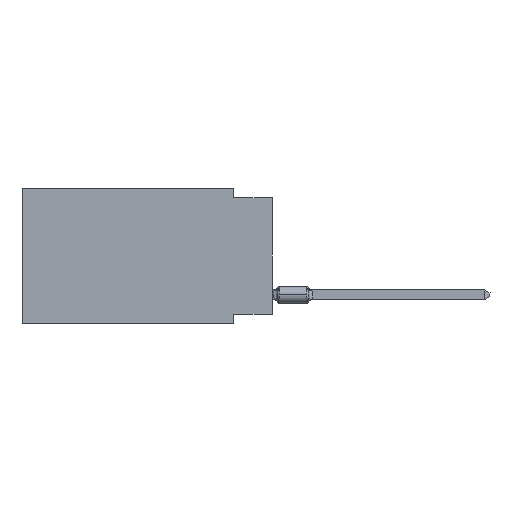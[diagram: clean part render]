
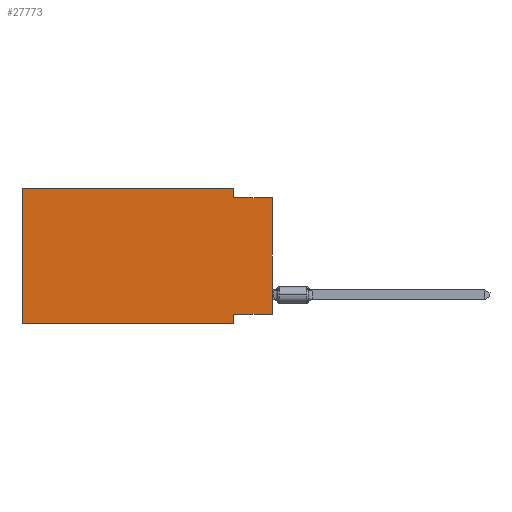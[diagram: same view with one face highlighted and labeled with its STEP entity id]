
A CAD part, left-side view. The second image highlights one B-rep face of the part: STEP entity #27773.
In plain terms, the highlighted planar face has unit normal (-1, 0, 0).
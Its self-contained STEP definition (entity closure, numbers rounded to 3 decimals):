
#157 = ORIENTED_EDGE ( 'NONE', *, *, #20566, .F. ) ;
#1232 = VERTEX_POINT ( 'NONE', #8478 ) ;
#1319 = VERTEX_POINT ( 'NONE', #1795 ) ;
#1593 = EDGE_CURVE ( 'NONE', #19388, #13219, #30711, .T. ) ;
#1795 = CARTESIAN_POINT ( 'NONE',  ( 0., 2.54, -8.255 ) ) ;
#1906 = DIRECTION ( 'NONE',  ( 0., -1., 0. ) ) ;
#2974 = LINE ( 'NONE', #7769, #18852 ) ;
#3166 = CARTESIAN_POINT ( 'NONE',  ( 0., 0., -0.635 ) ) ;
#3700 = LINE ( 'NONE', #13406, #22233 ) ;
#3973 = EDGE_CURVE ( 'NONE', #13219, #11547, #6130, .T. ) ;
#4017 = CARTESIAN_POINT ( 'NONE',  ( 0., 16.383, 0. ) ) ;
#4043 = AXIS2_PLACEMENT_3D ( 'NONE', #4017, #11180, #21385 ) ;
#4394 = LINE ( 'NONE', #12014, #19339 ) ;
#4934 = EDGE_CURVE ( 'NONE', #19388, #9634, #21191, .T. ) ;
#5345 = VERTEX_POINT ( 'NONE', #3166 ) ;
#5811 = VERTEX_POINT ( 'NONE', #7577 ) ;
#6130 = LINE ( 'NONE', #15852, #12876 ) ;
#6335 = CARTESIAN_POINT ( 'NONE',  ( 0., 16.383, 0. ) ) ;
#7226 = LINE ( 'NONE', #22345, #17469 ) ;
#7577 = CARTESIAN_POINT ( 'NONE',  ( 0., 0., -8.255 ) ) ;
#7591 = DIRECTION ( 'NONE',  ( 0., 0., 1. ) ) ;
#7677 = ORIENTED_EDGE ( 'NONE', *, *, #4934, .T. ) ;
#7769 = CARTESIAN_POINT ( 'NONE',  ( 0., 0., 0. ) ) ;
#7908 = CARTESIAN_POINT ( 'NONE',  ( 0., 2.54, -8.89 ) ) ;
#8305 = ORIENTED_EDGE ( 'NONE', *, *, #1593, .F. ) ;
#8478 = CARTESIAN_POINT ( 'NONE',  ( 0., 2.54, -0.635 ) ) ;
#8946 = PLANE ( 'NONE',  #4043 ) ;
#9634 = VERTEX_POINT ( 'NONE', #7908 ) ;
#9698 = EDGE_CURVE ( 'NONE', #5811, #5345, #2974, .T. ) ;
#10855 = DIRECTION ( 'NONE',  ( 0., -1., 0. ) ) ;
#10997 = ORIENTED_EDGE ( 'NONE', *, *, #27568, .F. ) ;
#11180 = DIRECTION ( 'NONE',  ( 1., 0., 0. ) ) ;
#11547 = VERTEX_POINT ( 'NONE', #21206 ) ;
#11580 = VECTOR ( 'NONE', #19209, 1000. ) ;
#12014 = CARTESIAN_POINT ( 'NONE',  ( 0., 2.54, -8.89 ) ) ;
#12876 = VECTOR ( 'NONE', #25576, 1000. ) ;
#13219 = VERTEX_POINT ( 'NONE', #17408 ) ;
#13406 = CARTESIAN_POINT ( 'NONE',  ( 0., 0., -0.635 ) ) ;
#14019 = CARTESIAN_POINT ( 'NONE',  ( 0., 16.383, -8.89 ) ) ;
#14486 = ORIENTED_EDGE ( 'NONE', *, *, #16283, .F. ) ;
#15090 = ORIENTED_EDGE ( 'NONE', *, *, #20014, .F. ) ;
#15160 = DIRECTION ( 'NONE',  ( 0., 0., -1. ) ) ;
#15852 = CARTESIAN_POINT ( 'NONE',  ( 0., 16.383, 0. ) ) ;
#16050 = DIRECTION ( 'NONE',  ( 0., 0., 1. ) ) ;
#16283 = EDGE_CURVE ( 'NONE', #1319, #9634, #4394, .T. ) ;
#17408 = CARTESIAN_POINT ( 'NONE',  ( 0., 16.383, 0. ) ) ;
#17469 = VECTOR ( 'NONE', #15160, 1000. ) ;
#17475 = ORIENTED_EDGE ( 'NONE', *, *, #3973, .F. ) ;
#18744 = LINE ( 'NONE', #28451, #11580 ) ;
#18852 = VECTOR ( 'NONE', #7591, 1000. ) ;
#19062 = CARTESIAN_POINT ( 'NONE',  ( 0., 16.383, -8.89 ) ) ;
#19209 = DIRECTION ( 'NONE',  ( 0., 1., 0. ) ) ;
#19339 = VECTOR ( 'NONE', #21592, 1000. ) ;
#19388 = VERTEX_POINT ( 'NONE', #19062 ) ;
#20014 = EDGE_CURVE ( 'NONE', #1232, #5345, #3700, .T. ) ;
#20566 = EDGE_CURVE ( 'NONE', #5811, #1319, #18744, .T. ) ;
#21071 = FACE_OUTER_BOUND ( 'NONE', #31429, .T. ) ;
#21191 = LINE ( 'NONE', #14019, #28073 ) ;
#21206 = CARTESIAN_POINT ( 'NONE',  ( 0., 2.54, 0. ) ) ;
#21385 = DIRECTION ( 'NONE',  ( 0., 0., -1. ) ) ;
#21592 = DIRECTION ( 'NONE',  ( 0., 0., -1. ) ) ;
#21718 = VECTOR ( 'NONE', #16050, 1000. ) ;
#22233 = VECTOR ( 'NONE', #10855, 1000. ) ;
#22345 = CARTESIAN_POINT ( 'NONE',  ( 0., 2.54, 0. ) ) ;
#25576 = DIRECTION ( 'NONE',  ( 0., -1., 0. ) ) ;
#27174 = ORIENTED_EDGE ( 'NONE', *, *, #9698, .T. ) ;
#27568 = EDGE_CURVE ( 'NONE', #11547, #1232, #7226, .T. ) ;
#27773 = ADVANCED_FACE ( 'NONE', ( #21071 ), #8946, .F. ) ;
#28073 = VECTOR ( 'NONE', #1906, 1000. ) ;
#28451 = CARTESIAN_POINT ( 'NONE',  ( 0., 0., -8.255 ) ) ;
#30711 = LINE ( 'NONE', #6335, #21718 ) ;
#31429 = EDGE_LOOP ( 'NONE', ( #27174, #15090, #10997, #17475, #8305, #7677, #14486, #157 ) ) ;
